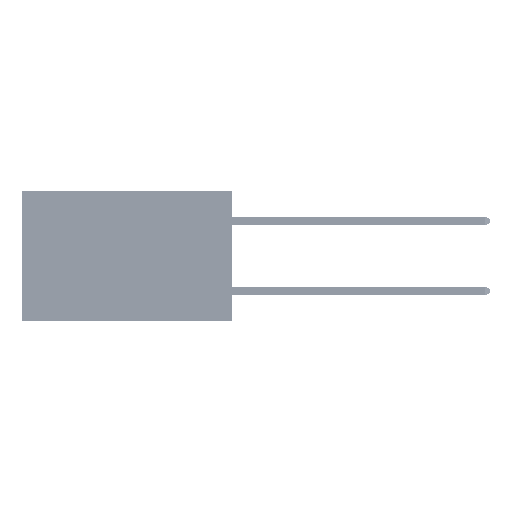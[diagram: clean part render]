
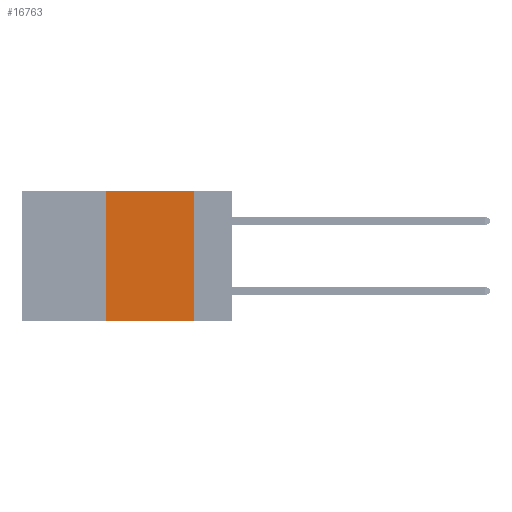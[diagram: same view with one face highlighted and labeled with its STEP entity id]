
A CAD part, left-side view. The second image highlights one B-rep face of the part: STEP entity #16763.
In plain terms, the highlighted planar face has unit normal (-1, 0, 0).
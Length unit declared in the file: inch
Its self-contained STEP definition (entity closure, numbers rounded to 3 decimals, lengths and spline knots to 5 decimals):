
#225 = CARTESIAN_POINT ( 'NONE',  ( 0., 0.11, -0.37 ) ) ;
#551 = CARTESIAN_POINT ( 'NONE',  ( 0., 0.6, -0.37 ) ) ;
#1283 = EDGE_CURVE ( 'NONE', #18164, #27966, #42551, .T. ) ;
#3213 = VERTEX_POINT ( 'NONE', #26759 ) ;
#4942 = DIRECTION ( 'NONE',  ( 0., 0., -1. ) ) ;
#9765 = LINE ( 'NONE', #37131, #37066 ) ;
#11626 = DIRECTION ( 'NONE',  ( 1., 0., 0. ) ) ;
#13120 = LINE ( 'NONE', #36482, #41162 ) ;
#13373 = VERTEX_POINT ( 'NONE', #37621 ) ;
#13859 = ORIENTED_EDGE ( 'NONE', *, *, #39162, .F. ) ;
#16763 = ADVANCED_FACE ( 'NONE', ( #38014 ), #34533, .F. ) ;
#18164 = VERTEX_POINT ( 'NONE', #41753 ) ;
#19020 = LINE ( 'NONE', #551, #37939 ) ;
#19411 = ORIENTED_EDGE ( 'NONE', *, *, #1283, .F. ) ;
#19517 = DIRECTION ( 'NONE',  ( 0., -1., 0. ) ) ;
#24094 = ORIENTED_EDGE ( 'NONE', *, *, #48524, .F. ) ;
#26759 = CARTESIAN_POINT ( 'NONE',  ( 0., 0.36, -0.37 ) ) ;
#27966 = VERTEX_POINT ( 'NONE', #225 ) ;
#30100 = AXIS2_PLACEMENT_3D ( 'NONE', #30821, #11626, #34288 ) ;
#30821 = CARTESIAN_POINT ( 'NONE',  ( 0., 0.6, 0. ) ) ;
#34288 = DIRECTION ( 'NONE',  ( 0., 0., -1. ) ) ;
#34533 = PLANE ( 'NONE',  #30100 ) ;
#36393 = DIRECTION ( 'NONE',  ( 0., 0., 1. ) ) ;
#36482 = CARTESIAN_POINT ( 'NONE',  ( 0., 0.6, 0. ) ) ;
#37066 = VECTOR ( 'NONE', #36393, 39.37008 ) ;
#37131 = CARTESIAN_POINT ( 'NONE',  ( 0., 0.36, 0. ) ) ;
#37621 = CARTESIAN_POINT ( 'NONE',  ( 0., 0.36, 0. ) ) ;
#37939 = VECTOR ( 'NONE', #19517, 39.37008 ) ;
#38014 = FACE_OUTER_BOUND ( 'NONE', #39901, .T. ) ;
#39162 = EDGE_CURVE ( 'NONE', #13373, #18164, #13120, .T. ) ;
#39901 = EDGE_LOOP ( 'NONE', ( #19411, #13859, #24094, #42699 ) ) ;
#39907 = EDGE_CURVE ( 'NONE', #3213, #27966, #19020, .T. ) ;
#40467 = DIRECTION ( 'NONE',  ( 0., -1., 0. ) ) ;
#41162 = VECTOR ( 'NONE', #40467, 39.37008 ) ;
#41753 = CARTESIAN_POINT ( 'NONE',  ( 0., 0.11, 0. ) ) ;
#42551 = LINE ( 'NONE', #45786, #45609 ) ;
#42699 = ORIENTED_EDGE ( 'NONE', *, *, #39907, .T. ) ;
#45609 = VECTOR ( 'NONE', #4942, 39.37008 ) ;
#45786 = CARTESIAN_POINT ( 'NONE',  ( 0., 0.11, 0. ) ) ;
#48524 = EDGE_CURVE ( 'NONE', #3213, #13373, #9765, .T. ) ;
